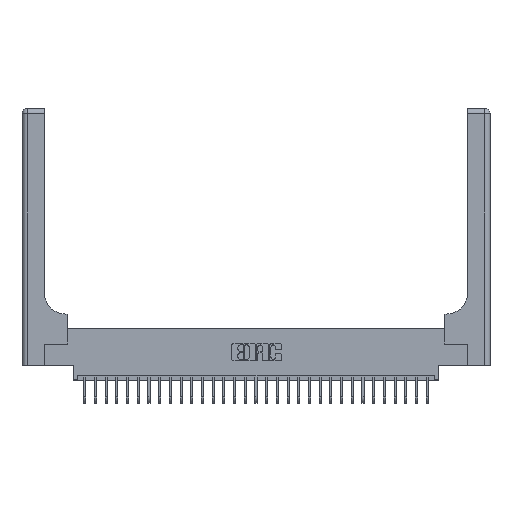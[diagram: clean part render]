
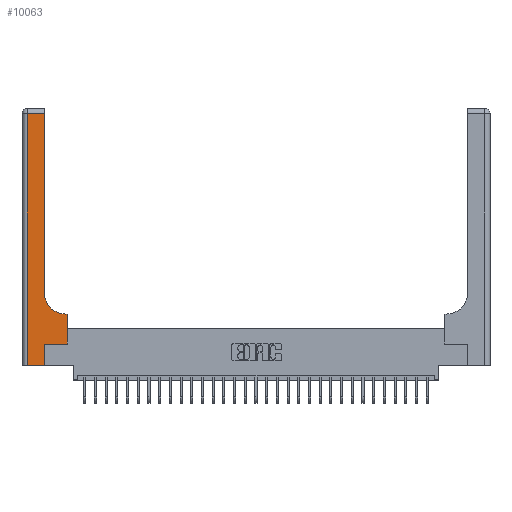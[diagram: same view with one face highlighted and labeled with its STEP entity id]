
A CAD part, top view. The second image highlights one B-rep face of the part: STEP entity #10063.
In plain terms, the highlighted planar face has unit normal (0, 0, 1).
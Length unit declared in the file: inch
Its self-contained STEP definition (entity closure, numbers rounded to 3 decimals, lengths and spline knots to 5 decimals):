
#16 = ORIENTED_EDGE ( 'NONE', *, *, #19261, .T. ) ;
#96 = LINE ( 'NONE', #1457, #16175 ) ;
#704 = EDGE_LOOP ( 'NONE', ( #17572, #22732, #15379, #6003, #16, #13034, #20159, #17316, #10584 ) ) ;
#1345 = LINE ( 'NONE', #24176, #11907 ) ;
#1457 = CARTESIAN_POINT ( 'NONE',  ( 0.265, 0., 0.37 ) ) ;
#1510 = CARTESIAN_POINT ( 'NONE',  ( 0.265, 0., 0.37 ) ) ;
#1796 = CARTESIAN_POINT ( 'NONE',  ( 0.06, 2.94, 0.37 ) ) ;
#1848 = EDGE_CURVE ( 'NONE', #25794, #19881, #19335, .T. ) ;
#1961 = LINE ( 'NONE', #18726, #12519 ) ;
#1990 = CARTESIAN_POINT ( 'NONE',  ( 0.265, 0.25, 0.37 ) ) ;
#2177 = EDGE_CURVE ( 'NONE', #19139, #9524, #22590, .T. ) ;
#2509 = CARTESIAN_POINT ( 'NONE',  ( 0.51, 0.6, 0.37 ) ) ;
#2785 = VERTEX_POINT ( 'NONE', #2509 ) ;
#3268 = LINE ( 'NONE', #1990, #26155 ) ;
#3328 = DIRECTION ( 'NONE',  ( 0., -1., 0. ) ) ;
#3719 = AXIS2_PLACEMENT_3D ( 'NONE', #16618, #4084, #18720 ) ;
#4027 = LINE ( 'NONE', #9748, #10955 ) ;
#4084 = DIRECTION ( 'NONE',  ( 0., 0., -1. ) ) ;
#5919 = VECTOR ( 'NONE', #25597, 39.37008 ) ;
#5930 = VERTEX_POINT ( 'NONE', #18567 ) ;
#5946 = CIRCLE ( 'NONE', #3719, 0.25 ) ;
#6003 = ORIENTED_EDGE ( 'NONE', *, *, #1848, .T. ) ;
#6040 = PLANE ( 'NONE',  #26553 ) ;
#6864 = CARTESIAN_POINT ( 'NONE',  ( 0., 2.94, 0.37 ) ) ;
#7298 = CARTESIAN_POINT ( 'NONE',  ( 0.528, 0.6, 0.37 ) ) ;
#7871 = DIRECTION ( 'NONE',  ( 0., 1., 0. ) ) ;
#8268 = VECTOR ( 'NONE', #12073, 39.37008 ) ;
#9518 = VERTEX_POINT ( 'NONE', #12206 ) ;
#9524 = VERTEX_POINT ( 'NONE', #1796 ) ;
#9703 = VECTOR ( 'NONE', #19205, 39.37008 ) ;
#9748 = CARTESIAN_POINT ( 'NONE',  ( 0.06, 3., 0.37 ) ) ;
#10063 = ADVANCED_FACE ( 'NONE', ( #18182 ), #6040, .F. ) ;
#10584 = ORIENTED_EDGE ( 'NONE', *, *, #15576, .T. ) ;
#10955 = VECTOR ( 'NONE', #3328, 39.37008 ) ;
#11583 = EDGE_CURVE ( 'NONE', #9518, #19139, #25014, .T. ) ;
#11907 = VECTOR ( 'NONE', #20001, 39.37008 ) ;
#12073 = DIRECTION ( 'NONE',  ( 1., 0., 0. ) ) ;
#12206 = CARTESIAN_POINT ( 'NONE',  ( 0.26, 0.85, 0.37 ) ) ;
#12260 = CARTESIAN_POINT ( 'NONE',  ( 0., 3., 0.37 ) ) ;
#12354 = DIRECTION ( 'NONE',  ( 0., 0., -1. ) ) ;
#12519 = VECTOR ( 'NONE', #14635, 39.37008 ) ;
#12643 = VERTEX_POINT ( 'NONE', #20515 ) ;
#13003 = CARTESIAN_POINT ( 'NONE',  ( 0.26, 3., 0.37 ) ) ;
#13034 = ORIENTED_EDGE ( 'NONE', *, *, #14494, .T. ) ;
#13141 = EDGE_CURVE ( 'NONE', #9524, #25794, #4027, .T. ) ;
#13673 = EDGE_CURVE ( 'NONE', #23713, #2785, #1345, .T. ) ;
#13676 = CARTESIAN_POINT ( 'NONE',  ( 0.26, 2.94, 0.37 ) ) ;
#14494 = EDGE_CURVE ( 'NONE', #12643, #5930, #3268, .T. ) ;
#14635 = DIRECTION ( 'NONE',  ( 0., 1., 0. ) ) ;
#15198 = EDGE_CURVE ( 'NONE', #5930, #23713, #1961, .T. ) ;
#15379 = ORIENTED_EDGE ( 'NONE', *, *, #13141, .T. ) ;
#15576 = EDGE_CURVE ( 'NONE', #2785, #9518, #5946, .T. ) ;
#16175 = VECTOR ( 'NONE', #7871, 39.37008 ) ;
#16618 = CARTESIAN_POINT ( 'NONE',  ( 0.51, 0.85, 0.37 ) ) ;
#16652 = DIRECTION ( 'NONE',  ( 1., 0., 0. ) ) ;
#17316 = ORIENTED_EDGE ( 'NONE', *, *, #13673, .T. ) ;
#17572 = ORIENTED_EDGE ( 'NONE', *, *, #11583, .T. ) ;
#18182 = FACE_OUTER_BOUND ( 'NONE', #704, .T. ) ;
#18567 = CARTESIAN_POINT ( 'NONE',  ( 0.528, 0.25, 0.37 ) ) ;
#18720 = DIRECTION ( 'NONE',  ( 1., 0., 0. ) ) ;
#18726 = CARTESIAN_POINT ( 'NONE',  ( 0.528, 0.25, 0.37 ) ) ;
#19139 = VERTEX_POINT ( 'NONE', #13676 ) ;
#19205 = DIRECTION ( 'NONE',  ( 0., 1., 0. ) ) ;
#19261 = EDGE_CURVE ( 'NONE', #19881, #12643, #96, .T. ) ;
#19335 = LINE ( 'NONE', #22466, #8268 ) ;
#19881 = VERTEX_POINT ( 'NONE', #1510 ) ;
#20001 = DIRECTION ( 'NONE',  ( -1., 0., 0. ) ) ;
#20159 = ORIENTED_EDGE ( 'NONE', *, *, #15198, .T. ) ;
#20515 = CARTESIAN_POINT ( 'NONE',  ( 0.265, 0.25, 0.37 ) ) ;
#22466 = CARTESIAN_POINT ( 'NONE',  ( 0., 0., 0.37 ) ) ;
#22590 = LINE ( 'NONE', #6864, #5919 ) ;
#22732 = ORIENTED_EDGE ( 'NONE', *, *, #2177, .T. ) ;
#23713 = VERTEX_POINT ( 'NONE', #7298 ) ;
#24176 = CARTESIAN_POINT ( 'NONE',  ( 0.26, 0.6, 0.37 ) ) ;
#24603 = CARTESIAN_POINT ( 'NONE',  ( 0.06, 0., 0.37 ) ) ;
#25014 = LINE ( 'NONE', #13003, #9703 ) ;
#25597 = DIRECTION ( 'NONE',  ( -1., 0., 0. ) ) ;
#25794 = VERTEX_POINT ( 'NONE', #24603 ) ;
#26155 = VECTOR ( 'NONE', #16652, 39.37008 ) ;
#26553 = AXIS2_PLACEMENT_3D ( 'NONE', #12260, #12354, #26872 ) ;
#26872 = DIRECTION ( 'NONE',  ( -1., 0., 0. ) ) ;
